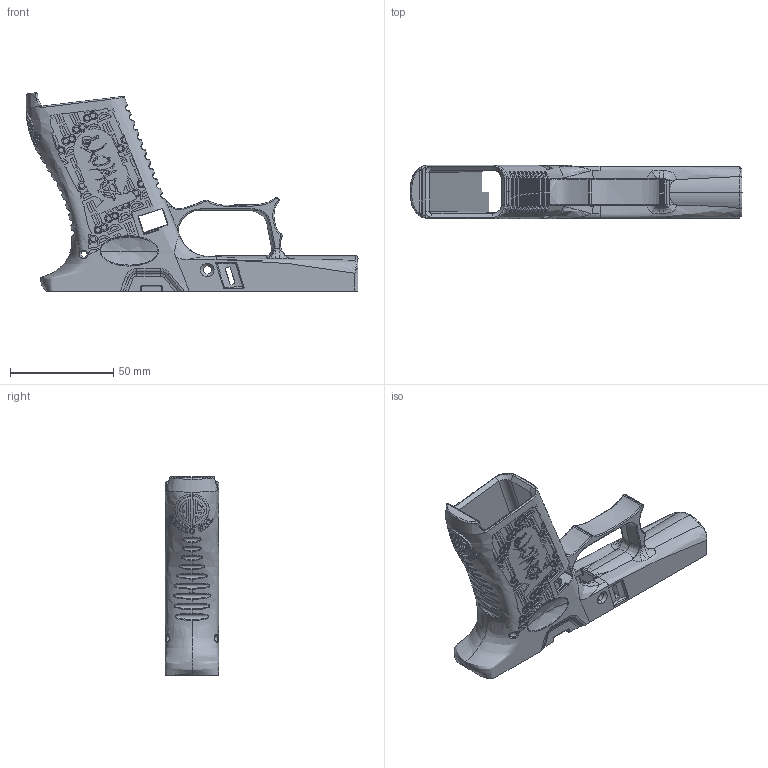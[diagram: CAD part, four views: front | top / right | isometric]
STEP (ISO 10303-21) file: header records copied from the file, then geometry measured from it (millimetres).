
FILE_DESCRIPTION (( 'STEP AP203' ), '1' );
FILE_NAME ('43X AWCY FDM.STEP', '2020-12-17T01:39:21', ( '' ), ( '' ), 'SwSTEP 2.0', 'SolidWorks 2016', '' );
FILE_SCHEMA (( 'CONFIG_CONTROL_DESIGN' ));
Products named in the file (1): 43X AWCY FDM
Bounding box: 160.56 x 25.9 x 95.92 mm (x, y, z)
Volume: 62514.8 mm3; surface area: 39911.4 mm2
Topology: 1 solids, 1 shells, 4295 faces, 12101 edges, 7924 vertices
Faces by surface type: plane 2365, cylinder 1326, bspline 564, torus 26, cone 12, sphere 2
Entity records: 340920 total; most frequent: CARTESIAN_POINT 240584, ORIENTED_EDGE 24130, DIRECTION 16080, EDGE_CURVE 12065, VERTEX_POINT 7924, LINE 5682, VECTOR 5682, AXIS2_PLACEMENT_3D 5199
